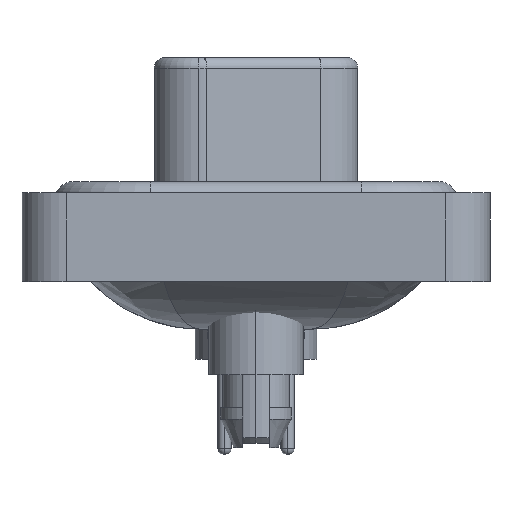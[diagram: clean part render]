
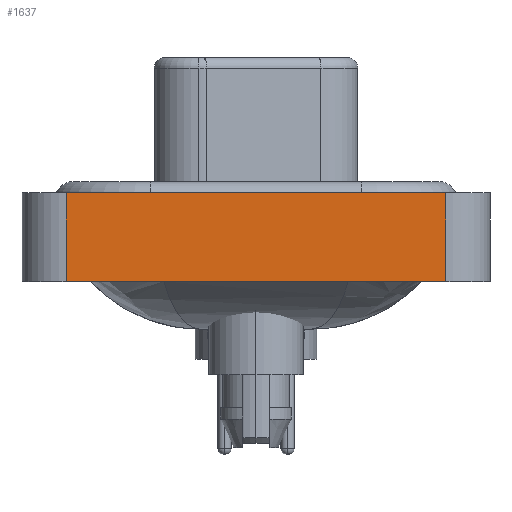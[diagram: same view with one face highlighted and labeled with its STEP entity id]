
A CAD part, left-side view. The second image highlights one B-rep face of the part: STEP entity #1637.
In plain terms, the highlighted planar face has unit normal (-1, 0, 0).
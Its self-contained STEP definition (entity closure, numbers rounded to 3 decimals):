
#222 = VECTOR ( 'NONE', #19020, 1000. ) ;
#598 = EDGE_CURVE ( 'NONE', #1339, #11805, #24125, .T. ) ;
#1339 = VERTEX_POINT ( 'NONE', #21739 ) ;
#1400 = ORIENTED_EDGE ( 'NONE', *, *, #7757, .T. ) ;
#1615 = VECTOR ( 'NONE', #19317, 1000. ) ;
#1637 = ADVANCED_FACE ( 'NONE', ( #23504 ), #4129, .T. ) ;
#4129 = PLANE ( 'NONE',  #10861 ) ;
#4324 = CARTESIAN_POINT ( 'NONE',  ( -7.35, 8.55, 0.4 ) ) ;
#4867 = CARTESIAN_POINT ( 'NONE',  ( -7.35, -8.55, -3.6 ) ) ;
#4936 = DIRECTION ( 'NONE',  ( 0., -1., 0. ) ) ;
#5191 = VERTEX_POINT ( 'NONE', #18452 ) ;
#5916 = LINE ( 'NONE', #6040, #1615 ) ;
#6040 = CARTESIAN_POINT ( 'NONE',  ( -7.35, -8.55, 0.4 ) ) ;
#7164 = VECTOR ( 'NONE', #13556, 1000. ) ;
#7757 = EDGE_CURVE ( 'NONE', #5191, #13377, #22220, .T. ) ;
#8396 = EDGE_CURVE ( 'NONE', #1339, #5191, #16030, .T. ) ;
#8944 = ORIENTED_EDGE ( 'NONE', *, *, #21270, .F. ) ;
#9115 = VECTOR ( 'NONE', #4936, 1000. ) ;
#9697 = CARTESIAN_POINT ( 'NONE',  ( -7.35, -8.55, -3.6 ) ) ;
#10861 = AXIS2_PLACEMENT_3D ( 'NONE', #9697, #11831, #13226 ) ;
#11805 = VERTEX_POINT ( 'NONE', #4324 ) ;
#11831 = DIRECTION ( 'NONE',  ( -1., 0., 0. ) ) ;
#13226 = DIRECTION ( 'NONE',  ( 0., 0., 1. ) ) ;
#13377 = VERTEX_POINT ( 'NONE', #20384 ) ;
#13556 = DIRECTION ( 'NONE',  ( 0., 0., 1. ) ) ;
#16030 = LINE ( 'NONE', #24199, #9115 ) ;
#18452 = CARTESIAN_POINT ( 'NONE',  ( -7.35, -8.55, -3.6 ) ) ;
#18764 = EDGE_LOOP ( 'NONE', ( #1400, #8944, #19758, #21313 ) ) ;
#19020 = DIRECTION ( 'NONE',  ( 0., 0., 1. ) ) ;
#19317 = DIRECTION ( 'NONE',  ( 0., -1., 0. ) ) ;
#19758 = ORIENTED_EDGE ( 'NONE', *, *, #598, .F. ) ;
#20384 = CARTESIAN_POINT ( 'NONE',  ( -7.35, -8.55, 0.4 ) ) ;
#21270 = EDGE_CURVE ( 'NONE', #11805, #13377, #5916, .T. ) ;
#21313 = ORIENTED_EDGE ( 'NONE', *, *, #8396, .T. ) ;
#21739 = CARTESIAN_POINT ( 'NONE',  ( -7.35, 8.55, -3.6 ) ) ;
#22215 = CARTESIAN_POINT ( 'NONE',  ( -7.35, 8.55, -3.6 ) ) ;
#22220 = LINE ( 'NONE', #4867, #222 ) ;
#23504 = FACE_OUTER_BOUND ( 'NONE', #18764, .T. ) ;
#24125 = LINE ( 'NONE', #22215, #7164 ) ;
#24199 = CARTESIAN_POINT ( 'NONE',  ( -7.35, -8.55, -3.6 ) ) ;
